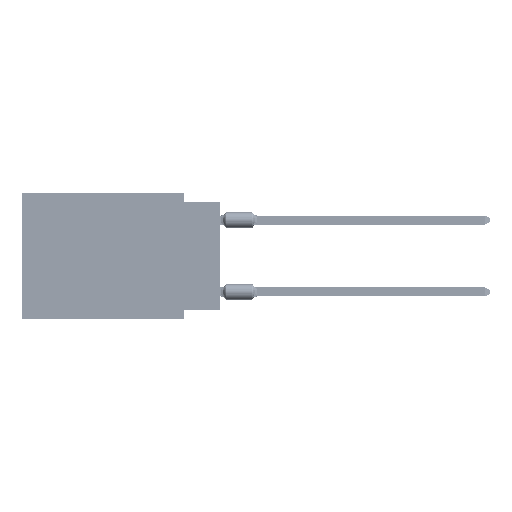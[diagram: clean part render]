
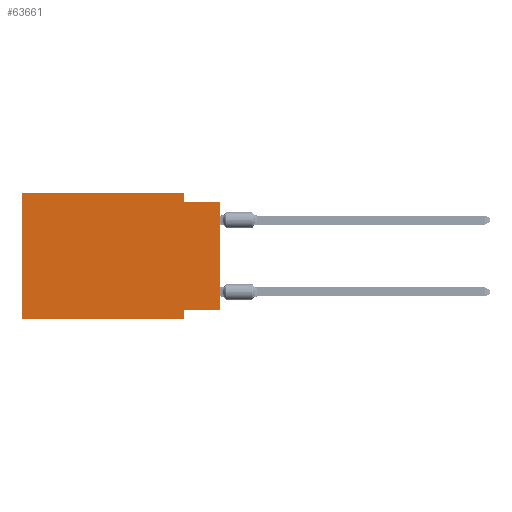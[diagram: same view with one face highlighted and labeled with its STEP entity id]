
A CAD part, left-side view. The second image highlights one B-rep face of the part: STEP entity #63661.
In plain terms, the highlighted planar face has unit normal (-1, 0, 0).
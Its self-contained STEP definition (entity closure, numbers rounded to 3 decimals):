
#547 = CARTESIAN_POINT ( 'NONE',  ( 0., 0., -8.255 ) ) ;
#1548 = DIRECTION ( 'NONE',  ( 0., -1., 0. ) ) ;
#3423 = ORIENTED_EDGE ( 'NONE', *, *, #52874, .F. ) ;
#3951 = CARTESIAN_POINT ( 'NONE',  ( 0., 13.97, -8.89 ) ) ;
#4535 = ORIENTED_EDGE ( 'NONE', *, *, #71331, .F. ) ;
#5025 = LINE ( 'NONE', #66115, #77508 ) ;
#5335 = EDGE_CURVE ( 'NONE', #46773, #76200, #42837, .T. ) ;
#5778 = VERTEX_POINT ( 'NONE', #25362 ) ;
#6120 = CARTESIAN_POINT ( 'NONE',  ( 0., 0., 0. ) ) ;
#7269 = CARTESIAN_POINT ( 'NONE',  ( 0., 2.54, 0. ) ) ;
#9404 = VERTEX_POINT ( 'NONE', #56481 ) ;
#10987 = EDGE_CURVE ( 'NONE', #63725, #42291, #5025, .T. ) ;
#12881 = AXIS2_PLACEMENT_3D ( 'NONE', #27832, #26257, #63867 ) ;
#13576 = VERTEX_POINT ( 'NONE', #29875 ) ;
#14392 = EDGE_LOOP ( 'NONE', ( #19004, #54629, #4535, #42536, #3423, #51681, #34049, #30682 ) ) ;
#14431 = VECTOR ( 'NONE', #25215, 1000. ) ;
#19004 = ORIENTED_EDGE ( 'NONE', *, *, #27452, .T. ) ;
#19164 = CARTESIAN_POINT ( 'NONE',  ( 0., 0., -0.635 ) ) ;
#19262 = DIRECTION ( 'NONE',  ( 0., 0., -1. ) ) ;
#19611 = VECTOR ( 'NONE', #34994, 1000. ) ;
#20063 = CARTESIAN_POINT ( 'NONE',  ( 0., 2.54, -8.89 ) ) ;
#20721 = LINE ( 'NONE', #547, #14431 ) ;
#25215 = DIRECTION ( 'NONE',  ( 0., 1., 0. ) ) ;
#25362 = CARTESIAN_POINT ( 'NONE',  ( 0., 2.54, -8.255 ) ) ;
#25835 = CARTESIAN_POINT ( 'NONE',  ( 0., 0., -0.635 ) ) ;
#26257 = DIRECTION ( 'NONE',  ( 1., 0., 0. ) ) ;
#26777 = EDGE_CURVE ( 'NONE', #9404, #78039, #38744, .T. ) ;
#27107 = EDGE_CURVE ( 'NONE', #5778, #42291, #35039, .T. ) ;
#27428 = FACE_OUTER_BOUND ( 'NONE', #14392, .T. ) ;
#27452 = EDGE_CURVE ( 'NONE', #13576, #76200, #79740, .T. ) ;
#27832 = CARTESIAN_POINT ( 'NONE',  ( 0., 13.97, 0. ) ) ;
#29875 = CARTESIAN_POINT ( 'NONE',  ( 0., 0., -8.255 ) ) ;
#30682 = ORIENTED_EDGE ( 'NONE', *, *, #39006, .F. ) ;
#34049 = ORIENTED_EDGE ( 'NONE', *, *, #27107, .F. ) ;
#34994 = DIRECTION ( 'NONE',  ( 0., 0., 1. ) ) ;
#35039 = LINE ( 'NONE', #20063, #38057 ) ;
#38057 = VECTOR ( 'NONE', #19262, 1000. ) ;
#38744 = LINE ( 'NONE', #50901, #52190 ) ;
#38782 = PLANE ( 'NONE',  #12881 ) ;
#39006 = EDGE_CURVE ( 'NONE', #13576, #5778, #20721, .T. ) ;
#40238 = VECTOR ( 'NONE', #78961, 1000. ) ;
#41841 = DIRECTION ( 'NONE',  ( 0., -1., 0. ) ) ;
#42291 = VERTEX_POINT ( 'NONE', #49503 ) ;
#42536 = ORIENTED_EDGE ( 'NONE', *, *, #26777, .F. ) ;
#42837 = LINE ( 'NONE', #25835, #68870 ) ;
#46773 = VERTEX_POINT ( 'NONE', #72347 ) ;
#48612 = DIRECTION ( 'NONE',  ( 0., 0., 1. ) ) ;
#48642 = LINE ( 'NONE', #7269, #40238 ) ;
#49503 = CARTESIAN_POINT ( 'NONE',  ( 0., 2.54, -8.89 ) ) ;
#50901 = CARTESIAN_POINT ( 'NONE',  ( 0., 13.97, 0. ) ) ;
#51681 = ORIENTED_EDGE ( 'NONE', *, *, #10987, .T. ) ;
#52190 = VECTOR ( 'NONE', #1548, 1000. ) ;
#52874 = EDGE_CURVE ( 'NONE', #63725, #9404, #65351, .T. ) ;
#54629 = ORIENTED_EDGE ( 'NONE', *, *, #5335, .F. ) ;
#56481 = CARTESIAN_POINT ( 'NONE',  ( 0., 13.97, 0. ) ) ;
#63661 = ADVANCED_FACE ( 'NONE', ( #27428 ), #38782, .F. ) ;
#63725 = VERTEX_POINT ( 'NONE', #3951 ) ;
#63867 = DIRECTION ( 'NONE',  ( 0., 0., -1. ) ) ;
#65351 = LINE ( 'NONE', #71421, #19611 ) ;
#66115 = CARTESIAN_POINT ( 'NONE',  ( 0., 13.97, -8.89 ) ) ;
#67932 = DIRECTION ( 'NONE',  ( 0., -1., 0. ) ) ;
#68870 = VECTOR ( 'NONE', #67932, 1000. ) ;
#69076 = VECTOR ( 'NONE', #48612, 1000. ) ;
#70804 = CARTESIAN_POINT ( 'NONE',  ( 0., 2.54, 0. ) ) ;
#71331 = EDGE_CURVE ( 'NONE', #78039, #46773, #48642, .T. ) ;
#71421 = CARTESIAN_POINT ( 'NONE',  ( 0., 13.97, 0. ) ) ;
#72347 = CARTESIAN_POINT ( 'NONE',  ( 0., 2.54, -0.635 ) ) ;
#76200 = VERTEX_POINT ( 'NONE', #19164 ) ;
#77508 = VECTOR ( 'NONE', #41841, 1000. ) ;
#78039 = VERTEX_POINT ( 'NONE', #70804 ) ;
#78961 = DIRECTION ( 'NONE',  ( 0., 0., -1. ) ) ;
#79740 = LINE ( 'NONE', #6120, #69076 ) ;
